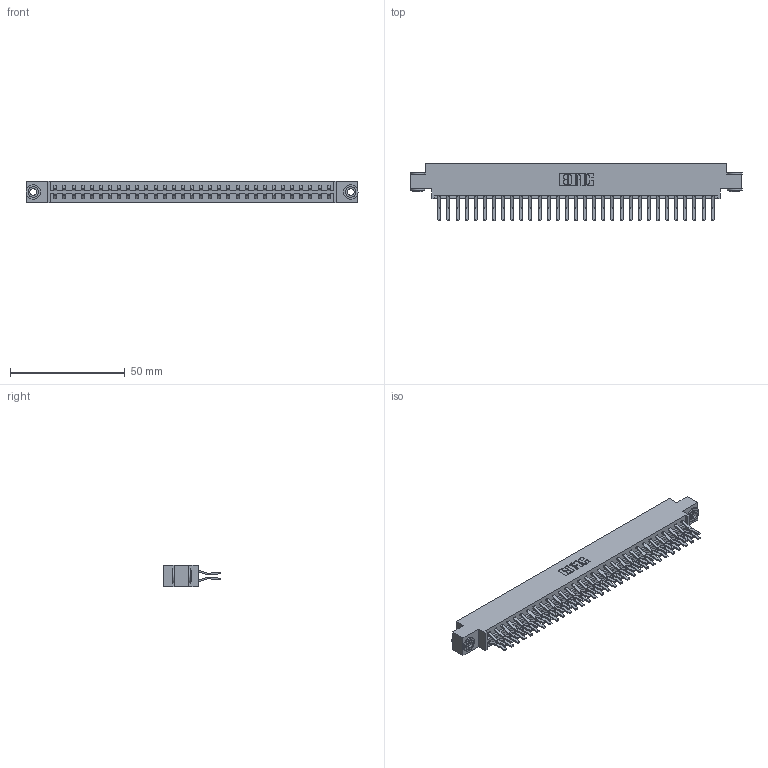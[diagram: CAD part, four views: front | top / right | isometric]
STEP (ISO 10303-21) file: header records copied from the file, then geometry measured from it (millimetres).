
FILE_DESCRIPTION (( 'STEP AP203' ), '1' );
FILE_NAME ('833-062-560-803.STEP', '2020-06-05T06:31:04', ( '' ), ( '' ), 'SwSTEP 2.0', 'SolidWorks 2020', '' );
FILE_SCHEMA (( 'CONFIG_CONTROL_DESIGN' ));
Length unit declared in the file: inch
Products named in the file (4): 833 Part_Offset - .156 Dia - TH; 345-292-001_560 Tail; 833-062-560-803; 345-250-002_345-250-002-102
Assembly tree (65 placements, depth 2):
  833-062-560-803
    833 Part_Offset - .156 Dia - TH
    345-292-001_560 Tail  x62
    345-250-002_345-250-002-102  x2
Bounding box: 144.37 x 24.78 x 9.4 mm (x, y, z)
Volume: 14834.8 mm3; surface area: 19021.3 mm2
Topology: 65 solids, 65 shells, 3504 faces, 10381 edges, 6834 vertices
Faces by surface type: plane 2316, cylinder 1180, cone 8
Entity records: 22236 total; most frequent: CARTESIAN_POINT 3677, ORIENTED_EDGE 3606, DIRECTION 3197, EDGE_CURVE 1803, LINE 1647, VECTOR 1647, VERTEX_POINT 1198, AXIS2_PLACEMENT_3D 775
